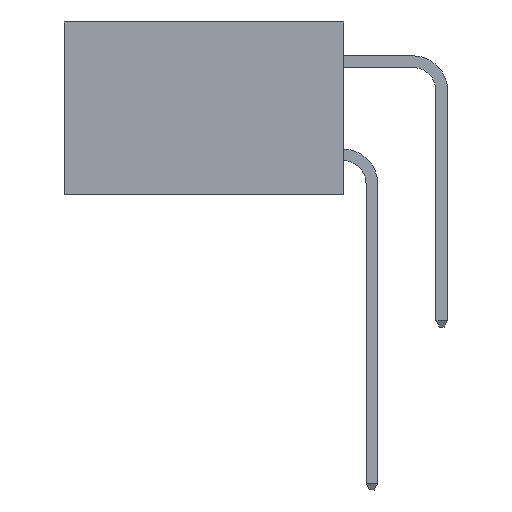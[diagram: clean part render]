
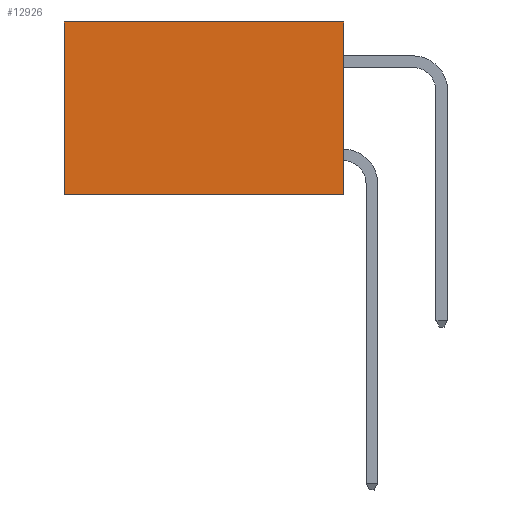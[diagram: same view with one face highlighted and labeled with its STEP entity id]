
A CAD part, left-side view. The second image highlights one B-rep face of the part: STEP entity #12926.
In plain terms, the highlighted planar face has unit normal (-1, 0, 0).
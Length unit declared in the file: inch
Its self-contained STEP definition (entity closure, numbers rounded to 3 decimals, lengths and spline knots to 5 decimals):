
#34 = CARTESIAN_POINT ( 'NONE',  ( 0.2615, 0.6, 0. ) ) ;
#651 = CARTESIAN_POINT ( 'NONE',  ( 0.2615, 0., 0. ) ) ;
#1486 = CARTESIAN_POINT ( 'NONE',  ( 0.2615, 0., -0.37 ) ) ;
#1746 = ORIENTED_EDGE ( 'NONE', *, *, #12794, .T. ) ;
#1928 = ORIENTED_EDGE ( 'NONE', *, *, #11171, .F. ) ;
#1993 = CARTESIAN_POINT ( 'NONE',  ( 0.2615, 0., -0.37 ) ) ;
#2239 = DIRECTION ( 'NONE',  ( 1., 0., 0. ) ) ;
#2265 = VECTOR ( 'NONE', #6720, 39.37008 ) ;
#2960 = LINE ( 'NONE', #1993, #9789 ) ;
#3681 = EDGE_CURVE ( 'NONE', #9707, #6057, #4445, .T. ) ;
#3962 = DIRECTION ( 'NONE',  ( 0., 0., -1. ) ) ;
#4237 = ORIENTED_EDGE ( 'NONE', *, *, #8153, .F. ) ;
#4431 = PLANE ( 'NONE',  #12189 ) ;
#4445 = LINE ( 'NONE', #11722, #2265 ) ;
#5231 = LINE ( 'NONE', #9493, #12389 ) ;
#6057 = VERTEX_POINT ( 'NONE', #34 ) ;
#6058 = DIRECTION ( 'NONE',  ( 0., 1., 0. ) ) ;
#6169 = DIRECTION ( 'NONE',  ( 0., 0., -1. ) ) ;
#6720 = DIRECTION ( 'NONE',  ( 0., 1., 0. ) ) ;
#6777 = CARTESIAN_POINT ( 'NONE',  ( 0.2615, 0.6, -0.37 ) ) ;
#7447 = VERTEX_POINT ( 'NONE', #1486 ) ;
#8153 = EDGE_CURVE ( 'NONE', #7447, #12416, #5231, .T. ) ;
#8809 = CARTESIAN_POINT ( 'NONE',  ( 0.2615, 0., -0.37 ) ) ;
#9493 = CARTESIAN_POINT ( 'NONE',  ( 0.2615, 0., -0.37 ) ) ;
#9707 = VERTEX_POINT ( 'NONE', #651 ) ;
#9789 = VECTOR ( 'NONE', #6169, 39.37008 ) ;
#11002 = ORIENTED_EDGE ( 'NONE', *, *, #3681, .T. ) ;
#11171 = EDGE_CURVE ( 'NONE', #9707, #7447, #2960, .T. ) ;
#11531 = VECTOR ( 'NONE', #3962, 39.37008 ) ;
#11712 = FACE_OUTER_BOUND ( 'NONE', #11885, .T. ) ;
#11722 = CARTESIAN_POINT ( 'NONE',  ( 0.2615, 0., 0. ) ) ;
#11885 = EDGE_LOOP ( 'NONE', ( #1746, #4237, #1928, #11002 ) ) ;
#11915 = DIRECTION ( 'NONE',  ( 0., 0., -1. ) ) ;
#12189 = AXIS2_PLACEMENT_3D ( 'NONE', #8809, #2239, #11915 ) ;
#12389 = VECTOR ( 'NONE', #6058, 39.37008 ) ;
#12416 = VERTEX_POINT ( 'NONE', #6777 ) ;
#12613 = CARTESIAN_POINT ( 'NONE',  ( 0.2615, 0.6, -0.37 ) ) ;
#12691 = LINE ( 'NONE', #12613, #11531 ) ;
#12794 = EDGE_CURVE ( 'NONE', #6057, #12416, #12691, .T. ) ;
#12926 = ADVANCED_FACE ( 'NONE', ( #11712 ), #4431, .F. ) ;
